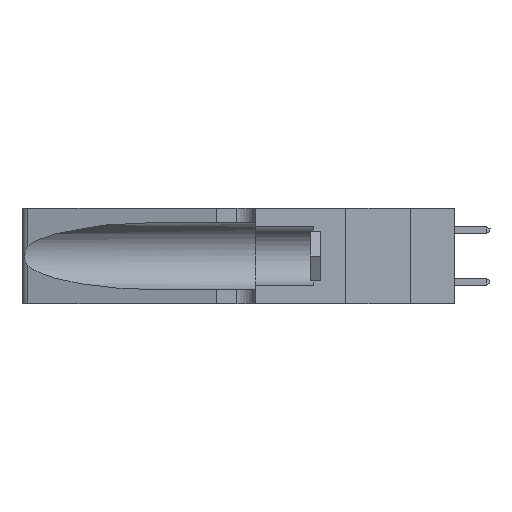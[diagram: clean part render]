
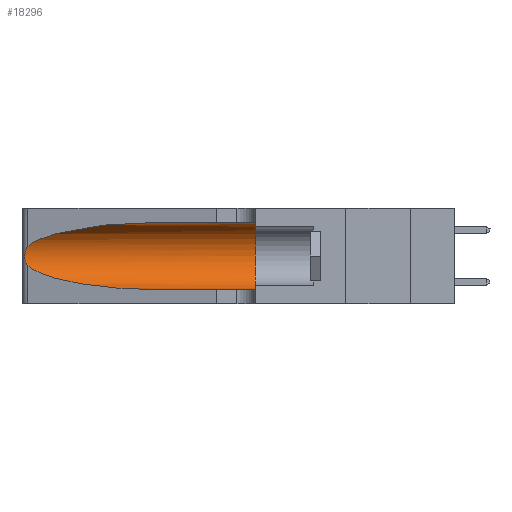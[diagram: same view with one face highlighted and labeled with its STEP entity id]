
A CAD part, left-side view. The second image highlights one B-rep face of the part: STEP entity #18296.
In plain terms, the highlighted cylindrical face has radius 3.308 mm (diameter 6.617 mm), a partial arc.
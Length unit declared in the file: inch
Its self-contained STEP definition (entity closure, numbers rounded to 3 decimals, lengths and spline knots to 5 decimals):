
#248 = EDGE_CURVE ( 'NONE', #9680, #3156, #9070, .T. ) ;
#455 = CYLINDRICAL_SURFACE ( 'NONE', #4932, 0.13025 ) ;
#486 = CARTESIAN_POINT ( 'NONE',  ( 0.25555, 1.22993, 0.14849 ) ) ;
#529 = CARTESIAN_POINT ( 'NONE',  ( 0.25639, 1.23186, 0.15144 ) ) ;
#693 = CARTESIAN_POINT ( 'NONE',  ( 0.25787, 1.23484, 0.2124 ) ) ;
#732 = CARTESIAN_POINT ( 'NONE',  ( 0.26075, 1.23896, 0.178 ) ) ;
#1283 = DIRECTION ( 'NONE',  ( 0., -1., 0. ) ) ;
#1640 =( BOUNDED_CURVE ( )  B_SPLINE_CURVE ( 3, ( #9352, #20373, #11583, #27017 ),
 .UNSPECIFIED., .F., .F. ) 
 B_SPLINE_CURVE_WITH_KNOTS ( ( 4, 4 ),
 ( 1.5708, 2.84003 ),
 .UNSPECIFIED. ) 
 CURVE ( )  GEOMETRIC_REPRESENTATION_ITEM ( )  RATIONAL_B_SPLINE_CURVE ( ( 1., 0.87, 0.87, 1. ) ) 
 REPRESENTATION_ITEM ( '' )  );
#1944 = CIRCLE ( 'NONE', #5192, 0.13025 ) ;
#3060 = CARTESIAN_POINT ( 'NONE',  ( 0.1305, 0.35, 0.185 ) ) ;
#3156 = VERTEX_POINT ( 'NONE', #15177 ) ;
#3180 = EDGE_CURVE ( 'NONE', #3156, #10450, #17201, .T. ) ;
#3442 = CARTESIAN_POINT ( 'NONE',  ( 0.1305, 1.61858, 0.31525 ) ) ;
#4015 = LINE ( 'NONE', #3442, #13828 ) ;
#4859 = ORIENTED_EDGE ( 'NONE', *, *, #16728, .F. ) ;
#4932 = AXIS2_PLACEMENT_3D ( 'NONE', #20124, #24547, #11327 ) ;
#5192 = AXIS2_PLACEMENT_3D ( 'NONE', #3060, #18663, #5332 ) ;
#5332 = DIRECTION ( 'NONE',  ( 0., 0., 1. ) ) ;
#6279 = EDGE_CURVE ( 'NONE', #10450, #18655, #19918, .T. ) ;
#9070 = B_SPLINE_CURVE_WITH_KNOTS ( 'NONE', 3,
 ( #20294, #20356, #20389, #693, #28231, #9463, #9427, #732, #20676, #20645, #20642, #529, #486, #20044 ),
 .UNSPECIFIED., .F., .F.,
 ( 4, 2, 2, 2, 2, 2, 4 ),
 ( 0., 0.00027, 0.00053, 0.00107, 0.0016, 0.00187, 0.00214 ),
 .UNSPECIFIED. ) ;
#9352 = CARTESIAN_POINT ( 'NONE',  ( 0.1305, 0.72297, 0.31525 ) ) ;
#9427 = CARTESIAN_POINT ( 'NONE',  ( 0.26075, 1.23896, 0.19203 ) ) ;
#9463 = CARTESIAN_POINT ( 'NONE',  ( 0.26018, 1.23835, 0.19895 ) ) ;
#9680 = VERTEX_POINT ( 'NONE', #23574 ) ;
#10450 = VERTEX_POINT ( 'NONE', #19509 ) ;
#10712 = EDGE_CURVE ( 'NONE', #27839, #9680, #1640, .T. ) ;
#10816 = CARTESIAN_POINT ( 'NONE',  ( 0.25487, 1.22718, 0.14631 ) ) ;
#11327 = DIRECTION ( 'NONE',  ( 0., 0., -1. ) ) ;
#11583 = CARTESIAN_POINT ( 'NONE',  ( 0.2373, 1.15595, 0.28018 ) ) ;
#13038 = CARTESIAN_POINT ( 'NONE',  ( 0.18966, 0.96281, 0.05475 ) ) ;
#13128 = CARTESIAN_POINT ( 'NONE',  ( 0.1305, 0.35, 0.31525 ) ) ;
#13828 = VECTOR ( 'NONE', #1283, 39.37008 ) ;
#13861 = CARTESIAN_POINT ( 'NONE',  ( 0.1305, 1.61858, 0.05475 ) ) ;
#14544 = VERTEX_POINT ( 'NONE', #13128 ) ;
#15177 = CARTESIAN_POINT ( 'NONE',  ( 0.25487, 1.22718, 0.14631 ) ) ;
#15338 = ORIENTED_EDGE ( 'NONE', *, *, #3180, .T. ) ;
#16728 = EDGE_CURVE ( 'NONE', #27839, #14544, #4015, .T. ) ;
#17201 =( BOUNDED_CURVE ( )  B_SPLINE_CURVE ( 3, ( #10816, #21838, #13038, #28462 ),
 .UNSPECIFIED., .F., .F. ) 
 B_SPLINE_CURVE_WITH_KNOTS ( ( 4, 4 ),
 ( 3.44316, 4.71239 ),
 .UNSPECIFIED. ) 
 CURVE ( )  GEOMETRIC_REPRESENTATION_ITEM ( )  RATIONAL_B_SPLINE_CURVE ( ( 1., 0.87, 0.87, 1. ) ) 
 REPRESENTATION_ITEM ( '' )  );
#18296 = ADVANCED_FACE ( 'NONE', ( #24818 ), #455, .F. ) ;
#18655 = VERTEX_POINT ( 'NONE', #21731 ) ;
#18663 = DIRECTION ( 'NONE',  ( 0., 1., 0. ) ) ;
#18980 = CARTESIAN_POINT ( 'NONE',  ( 0.1305, 0.72297, 0.31525 ) ) ;
#19087 = EDGE_LOOP ( 'NONE', ( #19133, #19825, #15338, #21221, #27070, #4859 ) ) ;
#19133 = ORIENTED_EDGE ( 'NONE', *, *, #10712, .T. ) ;
#19217 = VECTOR ( 'NONE', #22647, 39.37008 ) ;
#19509 = CARTESIAN_POINT ( 'NONE',  ( 0.1305, 0.72297, 0.05475 ) ) ;
#19825 = ORIENTED_EDGE ( 'NONE', *, *, #248, .T. ) ;
#19918 = LINE ( 'NONE', #13861, #19217 ) ;
#20044 = CARTESIAN_POINT ( 'NONE',  ( 0.25487, 1.22718, 0.14631 ) ) ;
#20124 = CARTESIAN_POINT ( 'NONE',  ( 0.1305, 1.61858, 0.185 ) ) ;
#20294 = CARTESIAN_POINT ( 'NONE',  ( 0.25487, 1.22718, 0.22369 ) ) ;
#20356 = CARTESIAN_POINT ( 'NONE',  ( 0.25555, 1.22994, 0.2215 ) ) ;
#20373 = CARTESIAN_POINT ( 'NONE',  ( 0.18966, 0.96281, 0.31525 ) ) ;
#20389 = CARTESIAN_POINT ( 'NONE',  ( 0.25639, 1.23184, 0.21858 ) ) ;
#20642 = CARTESIAN_POINT ( 'NONE',  ( 0.25789, 1.23486, 0.15765 ) ) ;
#20645 = CARTESIAN_POINT ( 'NONE',  ( 0.25856, 1.23593, 0.16098 ) ) ;
#20676 = CARTESIAN_POINT ( 'NONE',  ( 0.26017, 1.23833, 0.17102 ) ) ;
#21221 = ORIENTED_EDGE ( 'NONE', *, *, #6279, .T. ) ;
#21731 = CARTESIAN_POINT ( 'NONE',  ( 0.1305, 0.35, 0.05475 ) ) ;
#21838 = CARTESIAN_POINT ( 'NONE',  ( 0.2373, 1.15595, 0.08982 ) ) ;
#22647 = DIRECTION ( 'NONE',  ( 0., -1., 0. ) ) ;
#22727 = EDGE_CURVE ( 'NONE', #14544, #18655, #1944, .T. ) ;
#23574 = CARTESIAN_POINT ( 'NONE',  ( 0.25487, 1.22718, 0.22369 ) ) ;
#24547 = DIRECTION ( 'NONE',  ( 0., -1., 0. ) ) ;
#24818 = FACE_OUTER_BOUND ( 'NONE', #19087, .T. ) ;
#27017 = CARTESIAN_POINT ( 'NONE',  ( 0.25487, 1.22718, 0.22369 ) ) ;
#27070 = ORIENTED_EDGE ( 'NONE', *, *, #22727, .F. ) ;
#27839 = VERTEX_POINT ( 'NONE', #18980 ) ;
#28231 = CARTESIAN_POINT ( 'NONE',  ( 0.25854, 1.2359, 0.20912 ) ) ;
#28462 = CARTESIAN_POINT ( 'NONE',  ( 0.1305, 0.72297, 0.05475 ) ) ;
